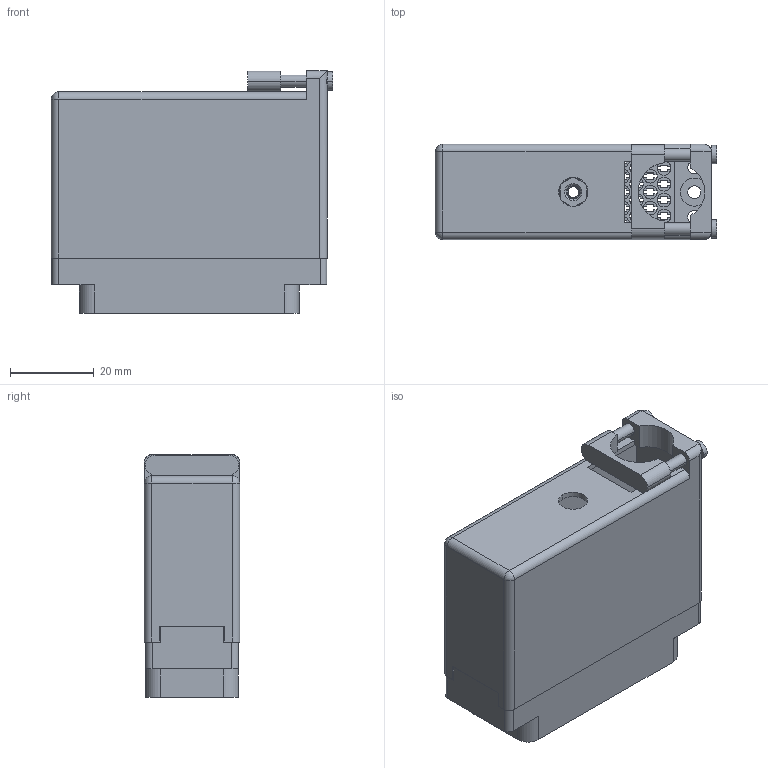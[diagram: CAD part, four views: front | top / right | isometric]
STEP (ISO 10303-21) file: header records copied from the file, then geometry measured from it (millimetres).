
FILE_DESCRIPTION (( 'STEP AP203' ), '1' );
FILE_NAME ('516-056-000-366.STEP', '2020-03-10T04:55:32', ( '' ), ( '' ), 'SwSTEP 2.0', 'SolidWorks 2016', '' );
FILE_SCHEMA (( 'CONFIG_CONTROL_DESIGN' ));
Length unit declared in the file: inch
Products named in the file (4): 516-056-000-366; 516-230-001_Metal - 056 Top Entry; 516 Plug Insulator_056; 516-252-035-100_516-252-035-100
Assembly tree (3 placements, depth 2):
  516-056-000-366
    516 Plug Insulator_056
    516-230-001_Metal - 056 Top Entry
    516-252-035-100_516-252-035-100
Bounding box: 67.31 x 22.83 x 58.12 mm (x, y, z)
Volume: 21979.6 mm3; surface area: 32348.2 mm2
Topology: 3 solids, 3 shells, 1334 faces, 3910 edges, 2598 vertices
Faces by surface type: plane 941, cylinder 373, cone 12, bspline 6, sphere 2
Entity records: 47252 total; most frequent: CARTESIAN_POINT 10334, ORIENTED_EDGE 7816, DIRECTION 7478, EDGE_CURVE 3908, VECTOR 2894, LINE 2894, VERTEX_POINT 2598, AXIS2_PLACEMENT_3D 2292
